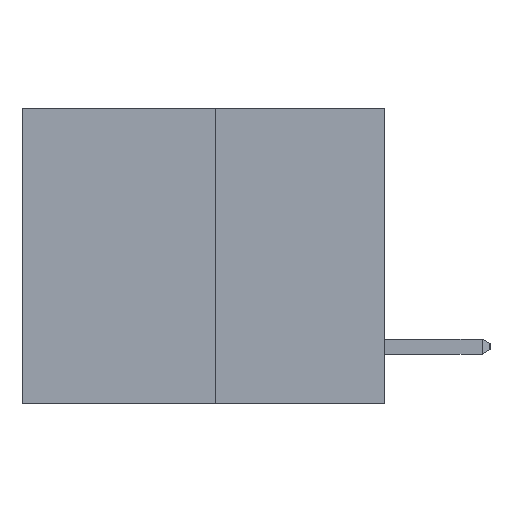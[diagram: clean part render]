
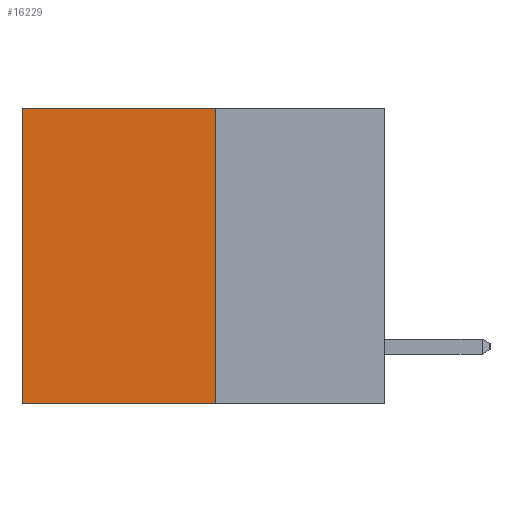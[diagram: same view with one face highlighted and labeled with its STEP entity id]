
A CAD part, left-side view. The second image highlights one B-rep face of the part: STEP entity #16229.
In plain terms, the highlighted planar face has unit normal (-1, 0, 0).
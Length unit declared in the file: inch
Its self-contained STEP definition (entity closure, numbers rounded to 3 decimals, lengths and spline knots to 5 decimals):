
#1331 = DIRECTION ( 'NONE',  ( 0., 0., -1. ) ) ;
#1786 = ORIENTED_EDGE ( 'NONE', *, *, #7443, .F. ) ;
#2105 = CARTESIAN_POINT ( 'NONE',  ( 0.3165, 0.6, -0.49 ) ) ;
#2338 = VERTEX_POINT ( 'NONE', #12457 ) ;
#7443 = EDGE_CURVE ( 'NONE', #10047, #10188, #13039, .T. ) ;
#7809 = CARTESIAN_POINT ( 'NONE',  ( 0.3165, 0.6, -0.49 ) ) ;
#8297 = AXIS2_PLACEMENT_3D ( 'NONE', #23025, #8406, #19771 ) ;
#8406 = DIRECTION ( 'NONE',  ( 1., 0., 0. ) ) ;
#9272 = ORIENTED_EDGE ( 'NONE', *, *, #10876, .T. ) ;
#10047 = VERTEX_POINT ( 'NONE', #12901 ) ;
#10181 = ORIENTED_EDGE ( 'NONE', *, *, #23857, .F. ) ;
#10188 = VERTEX_POINT ( 'NONE', #11158 ) ;
#10876 = EDGE_CURVE ( 'NONE', #2338, #20070, #18724, .T. ) ;
#11158 = CARTESIAN_POINT ( 'NONE',  ( 0.3165, 0.28, -0.49 ) ) ;
#11480 = DIRECTION ( 'NONE',  ( 0., 0., -1. ) ) ;
#11575 = EDGE_LOOP ( 'NONE', ( #9272, #10181, #1786, #23717 ) ) ;
#12119 = VECTOR ( 'NONE', #1331, 39.37008 ) ;
#12457 = CARTESIAN_POINT ( 'NONE',  ( 0.3165, 0.6, 0. ) ) ;
#12797 = EDGE_CURVE ( 'NONE', #10047, #2338, #20332, .T. ) ;
#12901 = CARTESIAN_POINT ( 'NONE',  ( 0.3165, 0.28, 0. ) ) ;
#13039 = LINE ( 'NONE', #19946, #12119 ) ;
#13118 = DIRECTION ( 'NONE',  ( 0., 1., 0. ) ) ;
#15088 = VECTOR ( 'NONE', #16267, 39.37008 ) ;
#15490 = VECTOR ( 'NONE', #11480, 39.37008 ) ;
#16229 = ADVANCED_FACE ( 'NONE', ( #20482 ), #21159, .F. ) ;
#16267 = DIRECTION ( 'NONE',  ( 0., 1., 0. ) ) ;
#18118 = VECTOR ( 'NONE', #13118, 39.37008 ) ;
#18232 = CARTESIAN_POINT ( 'NONE',  ( 0.3165, 0.28, 0. ) ) ;
#18724 = LINE ( 'NONE', #7809, #15490 ) ;
#19771 = DIRECTION ( 'NONE',  ( 0., 0., -1. ) ) ;
#19946 = CARTESIAN_POINT ( 'NONE',  ( 0.3165, 0.28, -0.49 ) ) ;
#20070 = VERTEX_POINT ( 'NONE', #2105 ) ;
#20332 = LINE ( 'NONE', #18232, #15088 ) ;
#20365 = CARTESIAN_POINT ( 'NONE',  ( 0.3165, 0.28, -0.49 ) ) ;
#20482 = FACE_OUTER_BOUND ( 'NONE', #11575, .T. ) ;
#21159 = PLANE ( 'NONE',  #8297 ) ;
#23025 = CARTESIAN_POINT ( 'NONE',  ( 0.3165, 0.28, -0.49 ) ) ;
#23646 = LINE ( 'NONE', #20365, #18118 ) ;
#23717 = ORIENTED_EDGE ( 'NONE', *, *, #12797, .T. ) ;
#23857 = EDGE_CURVE ( 'NONE', #10188, #20070, #23646, .T. ) ;
